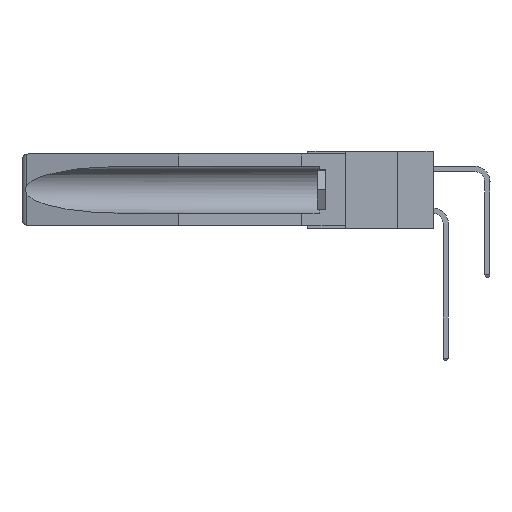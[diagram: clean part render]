
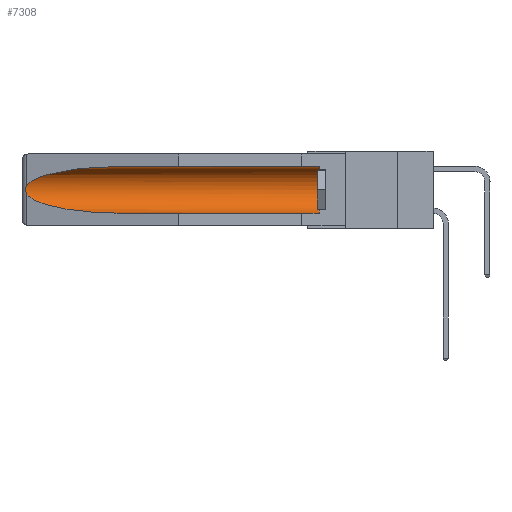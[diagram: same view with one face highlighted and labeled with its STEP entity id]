
A CAD part, left-side view. The second image highlights one B-rep face of the part: STEP entity #7308.
In plain terms, the highlighted cylindrical face has radius 2.857 mm (diameter 5.715 mm), a partial arc.
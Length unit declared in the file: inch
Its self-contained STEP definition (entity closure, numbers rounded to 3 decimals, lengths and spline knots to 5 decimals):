
#430 = VERTEX_POINT ( 'NONE', #16190 ) ;
#723 = ORIENTED_EDGE ( 'NONE', *, *, #4516, .T. ) ;
#831 = CARTESIAN_POINT ( 'NONE',  ( 0.155, 0.126, -0.059 ) ) ;
#1020 = ORIENTED_EDGE ( 'NONE', *, *, #17155, .T. ) ;
#1432 = CARTESIAN_POINT ( 'NONE',  ( 0.26655, 1.53094, -0.18657 ) ) ;
#1523 = AXIS2_PLACEMENT_3D ( 'NONE', #1725, #10126, #13452 ) ;
#1580 = CARTESIAN_POINT ( 'NONE',  ( 0.26537, 1.52718, -0.14972 ) ) ;
#1725 = CARTESIAN_POINT ( 'NONE',  ( 0.155, 0.126, -0.1715 ) ) ;
#1960 = ORIENTED_EDGE ( 'NONE', *, *, #21398, .T. ) ;
#2534 = AXIS2_PLACEMENT_3D ( 'NONE', #11514, #9867, #11584 ) ;
#3064 = EDGE_LOOP ( 'NONE', ( #1960, #10046, #1020, #21456, #10697, #723 ) ) ;
#3611 = LINE ( 'NONE', #6094, #20200 ) ;
#4516 = EDGE_CURVE ( 'NONE', #15966, #17979, #9016, .T. ) ;
#4838 = CARTESIAN_POINT ( 'NONE',  ( 0.26537, 1.52718, -0.19328 ) ) ;
#4974 = CARTESIAN_POINT ( 'NONE',  ( 0.25451, 1.48313, -0.09465 ) ) ;
#5587 = CARTESIAN_POINT ( 'NONE',  ( 0.21114, 1.30732, -0.059 ) ) ;
#6094 = CARTESIAN_POINT ( 'NONE',  ( 0.155, -0.30754, -0.284 ) ) ;
#6296 = CARTESIAN_POINT ( 'NONE',  ( 0.155, -0.30754, -0.059 ) ) ;
#6356 = CARTESIAN_POINT ( 'NONE',  ( 0.26654, 1.53092, -0.15636 ) ) ;
#6968 =( BOUNDED_CURVE ( )  B_SPLINE_CURVE ( 3, ( #16929, #15419, #8609, #18680 ),
 .UNSPECIFIED., .F., .F. ) 
 B_SPLINE_CURVE_WITH_KNOTS ( ( 4, 4 ),
 ( 0.1948, 1.5708 ),
 .UNSPECIFIED. ) 
 CURVE ( )  GEOMETRIC_REPRESENTATION_ITEM ( )  RATIONAL_B_SPLINE_CURVE ( ( 1., 0.848, 0.848, 1. ) ) 
 REPRESENTATION_ITEM ( '' )  );
#7308 = ADVANCED_FACE ( 'NONE', ( #15138 ), #14889, .F. ) ;
#7963 = CARTESIAN_POINT ( 'NONE',  ( 0.155, 1.07973, -0.059 ) ) ;
#8225 = CARTESIAN_POINT ( 'NONE',  ( 0.26597, 1.52961, -0.15275 ) ) ;
#8609 = CARTESIAN_POINT ( 'NONE',  ( 0.21114, 1.30732, -0.284 ) ) ;
#9016 = LINE ( 'NONE', #6296, #19132 ) ;
#9761 = CARTESIAN_POINT ( 'NONE',  ( 0.26537, 1.52718, -0.14972 ) ) ;
#9832 = CARTESIAN_POINT ( 'NONE',  ( 0.26597, 1.5296, -0.19026 ) ) ;
#9867 = DIRECTION ( 'NONE',  ( 0., 1., 0. ) ) ;
#9917 = EDGE_CURVE ( 'NONE', #13402, #14105, #3611, .T. ) ;
#10046 = ORIENTED_EDGE ( 'NONE', *, *, #17539, .T. ) ;
#10126 = DIRECTION ( 'NONE',  ( 0., -1., 0. ) ) ;
#10159 = CARTESIAN_POINT ( 'NONE',  ( 0.26537, 1.52718, -0.14972 ) ) ;
#10697 = ORIENTED_EDGE ( 'NONE', *, *, #16072, .T. ) ;
#11514 = CARTESIAN_POINT ( 'NONE',  ( 0.155, -0.30754, -0.1715 ) ) ;
#11584 = DIRECTION ( 'NONE',  ( 0., 0., 1. ) ) ;
#11969 = CIRCLE ( 'NONE', #1523, 0.1125 ) ;
#12788 = CARTESIAN_POINT ( 'NONE',  ( 0.155, 0.126, -0.284 ) ) ;
#12917 = VERTEX_POINT ( 'NONE', #10159 ) ;
#13402 = VERTEX_POINT ( 'NONE', #12788 ) ;
#13452 = DIRECTION ( 'NONE',  ( 0., 0., 1. ) ) ;
#13483 = B_SPLINE_CURVE_WITH_KNOTS ( 'NONE', 3,
 ( #1580, #8225, #6356, #17937, #19683, #19827, #17861, #1432, #9832, #4838 ),
 .UNSPECIFIED., .F., .F.,
 ( 4, 2, 2, 2, 4 ),
 ( 0., 0.00029, 0.00058, 0.00087, 0.00117 ),
 .UNSPECIFIED. ) ;
#14084 = CARTESIAN_POINT ( 'NONE',  ( 0.155, 1.07973, -0.284 ) ) ;
#14105 = VERTEX_POINT ( 'NONE', #14084 ) ;
#14889 = CYLINDRICAL_SURFACE ( 'NONE', #2534, 0.1125 ) ;
#15138 = FACE_OUTER_BOUND ( 'NONE', #3064, .T. ) ;
#15419 = CARTESIAN_POINT ( 'NONE',  ( 0.25451, 1.48313, -0.24835 ) ) ;
#15966 = VERTEX_POINT ( 'NONE', #831 ) ;
#16072 = EDGE_CURVE ( 'NONE', #13402, #15966, #11969, .T. ) ;
#16190 = CARTESIAN_POINT ( 'NONE',  ( 0.26537, 1.52718, -0.19328 ) ) ;
#16495 = CARTESIAN_POINT ( 'NONE',  ( 0.155, 1.07973, -0.059 ) ) ;
#16929 = CARTESIAN_POINT ( 'NONE',  ( 0.26537, 1.52718, -0.19328 ) ) ;
#17155 = EDGE_CURVE ( 'NONE', #430, #14105, #6968, .T. ) ;
#17539 = EDGE_CURVE ( 'NONE', #12917, #430, #13483, .T. ) ;
#17861 = CARTESIAN_POINT ( 'NONE',  ( 0.2673, 1.53269, -0.17917 ) ) ;
#17937 = CARTESIAN_POINT ( 'NONE',  ( 0.2673, 1.5327, -0.16383 ) ) ;
#17979 = VERTEX_POINT ( 'NONE', #7963 ) ;
#18680 = CARTESIAN_POINT ( 'NONE',  ( 0.155, 1.07973, -0.284 ) ) ;
#19132 = VECTOR ( 'NONE', #21352, 39.37008 ) ;
#19346 = DIRECTION ( 'NONE',  ( 0., 1., 0. ) ) ;
#19683 = CARTESIAN_POINT ( 'NONE',  ( 0.2675, 1.53308, -0.16763 ) ) ;
#19827 = CARTESIAN_POINT ( 'NONE',  ( 0.2675, 1.53308, -0.17534 ) ) ;
#20200 = VECTOR ( 'NONE', #19346, 39.37008 ) ;
#20528 =( BOUNDED_CURVE ( )  B_SPLINE_CURVE ( 3, ( #16495, #5587, #4974, #9761 ),
 .UNSPECIFIED., .F., .F. ) 
 B_SPLINE_CURVE_WITH_KNOTS ( ( 4, 4 ),
 ( 4.71239, 6.08839 ),
 .UNSPECIFIED. ) 
 CURVE ( )  GEOMETRIC_REPRESENTATION_ITEM ( )  RATIONAL_B_SPLINE_CURVE ( ( 1., 0.848, 0.848, 1. ) ) 
 REPRESENTATION_ITEM ( '' )  );
#21352 = DIRECTION ( 'NONE',  ( 0., 1., 0. ) ) ;
#21398 = EDGE_CURVE ( 'NONE', #17979, #12917, #20528, .T. ) ;
#21456 = ORIENTED_EDGE ( 'NONE', *, *, #9917, .F. ) ;
